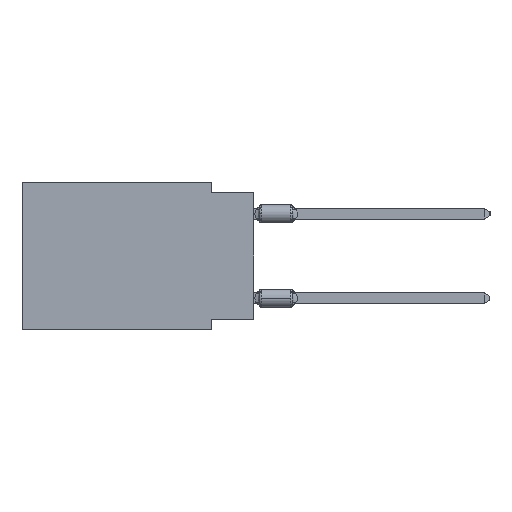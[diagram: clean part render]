
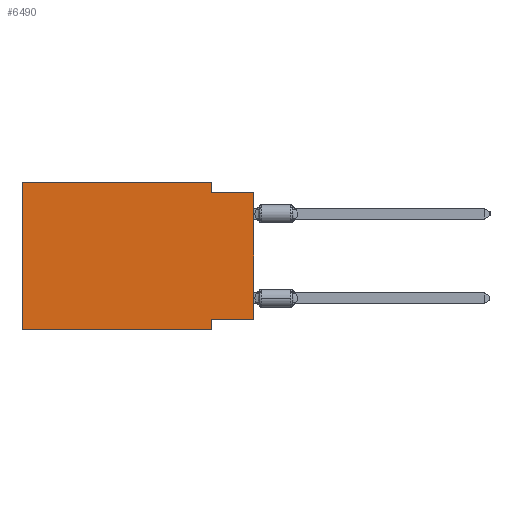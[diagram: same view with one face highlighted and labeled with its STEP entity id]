
A CAD part, left-side view. The second image highlights one B-rep face of the part: STEP entity #6490.
In plain terms, the highlighted planar face has unit normal (-1, 0, 0).
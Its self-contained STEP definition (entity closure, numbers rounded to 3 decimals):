
#252 = VECTOR ( 'NONE', #14826, 1000. ) ;
#545 = ORIENTED_EDGE ( 'NONE', *, *, #19398, .F. ) ;
#2513 = AXIS2_PLACEMENT_3D ( 'NONE', #10558, #8177, #10423 ) ;
#2709 = ORIENTED_EDGE ( 'NONE', *, *, #6176, .F. ) ;
#2874 = CARTESIAN_POINT ( 'NONE',  ( 0., 0., -8.255 ) ) ;
#2959 = ORIENTED_EDGE ( 'NONE', *, *, #17827, .F. ) ;
#3864 = DIRECTION ( 'NONE',  ( 0., -1., 0. ) ) ;
#3999 = CARTESIAN_POINT ( 'NONE',  ( 0., 0., -8.255 ) ) ;
#4790 = LINE ( 'NONE', #13374, #9788 ) ;
#4802 = VECTOR ( 'NONE', #5849, 1000. ) ;
#5849 = DIRECTION ( 'NONE',  ( 0., -1., 0. ) ) ;
#6065 = VERTEX_POINT ( 'NONE', #10593 ) ;
#6176 = EDGE_CURVE ( 'NONE', #23270, #26022, #23282, .T. ) ;
#6226 = DIRECTION ( 'NONE',  ( 0., -1., 0. ) ) ;
#6490 = ADVANCED_FACE ( 'NONE', ( #7767 ), #24932, .F. ) ;
#6912 = LINE ( 'NONE', #27119, #13825 ) ;
#7688 = CARTESIAN_POINT ( 'NONE',  ( 0., 13.97, -8.89 ) ) ;
#7767 = FACE_OUTER_BOUND ( 'NONE', #10012, .T. ) ;
#8154 = VECTOR ( 'NONE', #6226, 1000. ) ;
#8177 = DIRECTION ( 'NONE',  ( 1., 0., 0. ) ) ;
#8322 = DIRECTION ( 'NONE',  ( 0., 0., 1. ) ) ;
#8355 = VECTOR ( 'NONE', #3864, 1000. ) ;
#8877 = VERTEX_POINT ( 'NONE', #25876 ) ;
#9069 = VERTEX_POINT ( 'NONE', #18542 ) ;
#9437 = EDGE_CURVE ( 'NONE', #6065, #8877, #16673, .T. ) ;
#9788 = VECTOR ( 'NONE', #16030, 1000. ) ;
#10012 = EDGE_LOOP ( 'NONE', ( #10401, #11688, #2959, #14755, #545, #20944, #23489, #2709 ) ) ;
#10393 = CARTESIAN_POINT ( 'NONE',  ( 0., 2.54, -8.255 ) ) ;
#10401 = ORIENTED_EDGE ( 'NONE', *, *, #19278, .T. ) ;
#10423 = DIRECTION ( 'NONE',  ( 0., 0., -1. ) ) ;
#10558 = CARTESIAN_POINT ( 'NONE',  ( 0., 13.97, 0. ) ) ;
#10593 = CARTESIAN_POINT ( 'NONE',  ( 0., 13.97, 0. ) ) ;
#11688 = ORIENTED_EDGE ( 'NONE', *, *, #26832, .F. ) ;
#12973 = CARTESIAN_POINT ( 'NONE',  ( 0., 0., 0. ) ) ;
#13374 = CARTESIAN_POINT ( 'NONE',  ( 0., 2.54, 0. ) ) ;
#13403 = VERTEX_POINT ( 'NONE', #14957 ) ;
#13825 = VECTOR ( 'NONE', #22106, 1000. ) ;
#14755 = ORIENTED_EDGE ( 'NONE', *, *, #9437, .F. ) ;
#14826 = DIRECTION ( 'NONE',  ( 0., 1., 0. ) ) ;
#14939 = LINE ( 'NONE', #12973, #25969 ) ;
#14957 = CARTESIAN_POINT ( 'NONE',  ( 0., 13.97, -8.89 ) ) ;
#15425 = VERTEX_POINT ( 'NONE', #23589 ) ;
#16030 = DIRECTION ( 'NONE',  ( 0., 0., -1. ) ) ;
#16433 = VECTOR ( 'NONE', #17097, 1000. ) ;
#16673 = LINE ( 'NONE', #27225, #8355 ) ;
#17097 = DIRECTION ( 'NONE',  ( 0., 0., -1. ) ) ;
#17827 = EDGE_CURVE ( 'NONE', #8877, #15425, #4790, .T. ) ;
#18542 = CARTESIAN_POINT ( 'NONE',  ( 0., 0., -0.635 ) ) ;
#19278 = EDGE_CURVE ( 'NONE', #23270, #9069, #14939, .T. ) ;
#19398 = EDGE_CURVE ( 'NONE', #13403, #6065, #6912, .T. ) ;
#19443 = LINE ( 'NONE', #25508, #8154 ) ;
#20097 = EDGE_CURVE ( 'NONE', #26022, #22332, #23710, .T. ) ;
#20125 = CARTESIAN_POINT ( 'NONE',  ( 0., 2.54, -8.89 ) ) ;
#20944 = ORIENTED_EDGE ( 'NONE', *, *, #24459, .T. ) ;
#21734 = CARTESIAN_POINT ( 'NONE',  ( 0., 2.54, -8.89 ) ) ;
#22106 = DIRECTION ( 'NONE',  ( 0., 0., 1. ) ) ;
#22332 = VERTEX_POINT ( 'NONE', #20125 ) ;
#23270 = VERTEX_POINT ( 'NONE', #2874 ) ;
#23282 = LINE ( 'NONE', #3999, #252 ) ;
#23489 = ORIENTED_EDGE ( 'NONE', *, *, #20097, .F. ) ;
#23589 = CARTESIAN_POINT ( 'NONE',  ( 0., 2.54, -0.635 ) ) ;
#23710 = LINE ( 'NONE', #21734, #16433 ) ;
#24459 = EDGE_CURVE ( 'NONE', #13403, #22332, #24858, .T. ) ;
#24858 = LINE ( 'NONE', #7688, #4802 ) ;
#24932 = PLANE ( 'NONE',  #2513 ) ;
#25508 = CARTESIAN_POINT ( 'NONE',  ( 0., 0., -0.635 ) ) ;
#25876 = CARTESIAN_POINT ( 'NONE',  ( 0., 2.54, 0. ) ) ;
#25969 = VECTOR ( 'NONE', #8322, 1000. ) ;
#26022 = VERTEX_POINT ( 'NONE', #10393 ) ;
#26832 = EDGE_CURVE ( 'NONE', #15425, #9069, #19443, .T. ) ;
#27119 = CARTESIAN_POINT ( 'NONE',  ( 0., 13.97, 0. ) ) ;
#27225 = CARTESIAN_POINT ( 'NONE',  ( 0., 13.97, 0. ) ) ;
